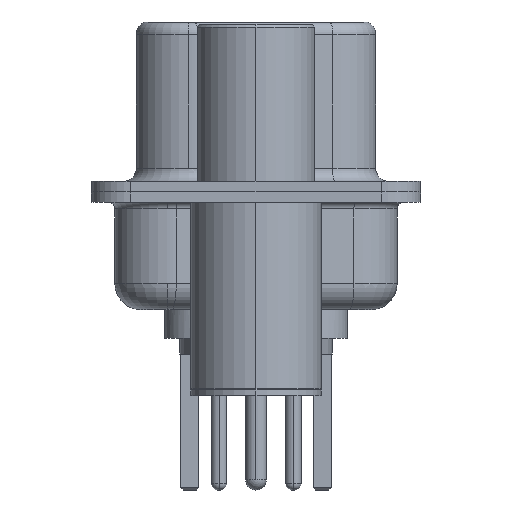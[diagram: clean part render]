
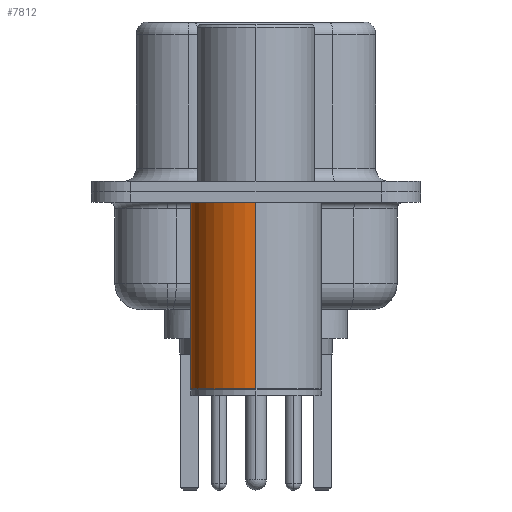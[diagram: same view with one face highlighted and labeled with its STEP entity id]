
A CAD part, left-side view. The second image highlights one B-rep face of the part: STEP entity #7812.
In plain terms, the highlighted cylindrical face has radius 2.5 mm (diameter 5 mm), a partial arc.
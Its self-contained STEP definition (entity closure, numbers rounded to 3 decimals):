
#317 = DIRECTION ( 'NONE',  ( 1., 0., 0. ) ) ;
#804 = EDGE_LOOP ( 'NONE', ( #11792, #24231, #14474, #23150 ) ) ;
#1772 = DIRECTION ( 'NONE',  ( 0., 0., 1. ) ) ;
#2907 = VERTEX_POINT ( 'NONE', #16259 ) ;
#5174 = CYLINDRICAL_SURFACE ( 'NONE', #7281, 2.5 ) ;
#5979 = VERTEX_POINT ( 'NONE', #19197 ) ;
#6586 = CARTESIAN_POINT ( 'NONE',  ( 0., 0., -7.525 ) ) ;
#7281 = AXIS2_PLACEMENT_3D ( 'NONE', #14228, #1772, #24493 ) ;
#7812 = ADVANCED_FACE ( 'NONE', ( #21496 ), #5174, .T. ) ;
#8065 = DIRECTION ( 'NONE',  ( 0., 0., 1. ) ) ;
#8624 = DIRECTION ( 'NONE',  ( 1., 0., 0. ) ) ;
#11406 = CARTESIAN_POINT ( 'NONE',  ( -2.5, 0., -0.4 ) ) ;
#11792 = ORIENTED_EDGE ( 'NONE', *, *, #17589, .T. ) ;
#11985 = AXIS2_PLACEMENT_3D ( 'NONE', #25144, #12776, #317 ) ;
#12776 = DIRECTION ( 'NONE',  ( 0., 0., 1. ) ) ;
#13687 = EDGE_CURVE ( 'NONE', #20137, #14565, #26762, .T. ) ;
#14228 = CARTESIAN_POINT ( 'NONE',  ( 0., 0., 0.581 ) ) ;
#14429 = CIRCLE ( 'NONE', #26751, 2.5 ) ;
#14474 = ORIENTED_EDGE ( 'NONE', *, *, #22423, .F. ) ;
#14565 = VERTEX_POINT ( 'NONE', #11406 ) ;
#14954 = CARTESIAN_POINT ( 'NONE',  ( -2.5, 0., 0.581 ) ) ;
#15552 = CARTESIAN_POINT ( 'NONE',  ( -2.5, 0., -7.525 ) ) ;
#15836 = VECTOR ( 'NONE', #19300, 1000. ) ;
#16259 = CARTESIAN_POINT ( 'NONE',  ( 2.5, 0., -7.525 ) ) ;
#16480 = VECTOR ( 'NONE', #8065, 1000. ) ;
#17589 = EDGE_CURVE ( 'NONE', #2907, #20137, #14429, .T. ) ;
#19197 = CARTESIAN_POINT ( 'NONE',  ( 2.5, 0., -0.4 ) ) ;
#19300 = DIRECTION ( 'NONE',  ( 0., 0., 1. ) ) ;
#20137 = VERTEX_POINT ( 'NONE', #15552 ) ;
#20899 = DIRECTION ( 'NONE',  ( 0., 0., 1. ) ) ;
#21496 = FACE_OUTER_BOUND ( 'NONE', #804, .T. ) ;
#22423 = EDGE_CURVE ( 'NONE', #5979, #14565, #26156, .T. ) ;
#22450 = CARTESIAN_POINT ( 'NONE',  ( 2.5, 0., 0.581 ) ) ;
#23057 = EDGE_CURVE ( 'NONE', #2907, #5979, #26131, .T. ) ;
#23150 = ORIENTED_EDGE ( 'NONE', *, *, #23057, .F. ) ;
#24231 = ORIENTED_EDGE ( 'NONE', *, *, #13687, .T. ) ;
#24493 = DIRECTION ( 'NONE',  ( 1., 0., 0. ) ) ;
#25144 = CARTESIAN_POINT ( 'NONE',  ( 0., 0., -0.4 ) ) ;
#26131 = LINE ( 'NONE', #22450, #16480 ) ;
#26156 = CIRCLE ( 'NONE', #11985, 2.5 ) ;
#26751 = AXIS2_PLACEMENT_3D ( 'NONE', #6586, #20899, #8624 ) ;
#26762 = LINE ( 'NONE', #14954, #15836 ) ;
